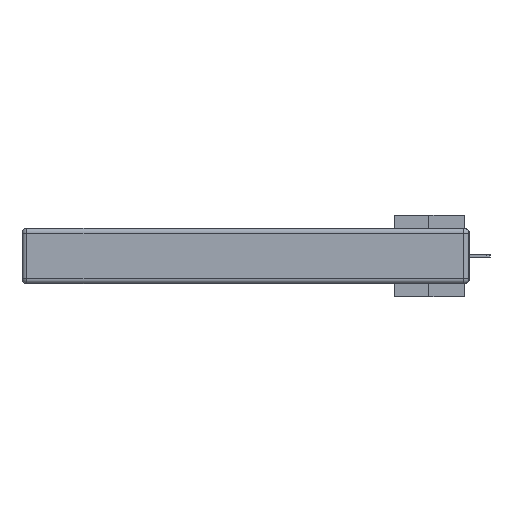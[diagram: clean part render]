
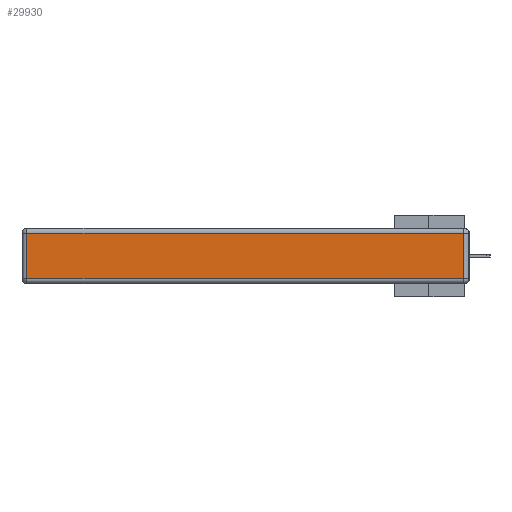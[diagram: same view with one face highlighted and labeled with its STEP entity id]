
A CAD part, left-side view. The second image highlights one B-rep face of the part: STEP entity #29930.
In plain terms, the highlighted planar face has unit normal (-1, 0, 0).
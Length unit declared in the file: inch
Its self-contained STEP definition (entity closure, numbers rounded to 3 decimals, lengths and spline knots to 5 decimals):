
#734 = LINE ( 'NONE', #21843, #33601 ) ;
#1146 = DIRECTION ( 'NONE',  ( 0., 0., -1. ) ) ;
#1558 = CARTESIAN_POINT ( 'NONE',  ( 0., 2.75, -0.03 ) ) ;
#3517 = EDGE_CURVE ( 'NONE', #15699, #11347, #24977, .T. ) ;
#5664 = EDGE_CURVE ( 'NONE', #13278, #15699, #734, .T. ) ;
#7889 = CARTESIAN_POINT ( 'NONE',  ( 0., 0.03, -0.313 ) ) ;
#8790 = EDGE_CURVE ( 'NONE', #21641, #13278, #31263, .T. ) ;
#10204 = DIRECTION ( 'NONE',  ( -1., 0., 0. ) ) ;
#11347 = VERTEX_POINT ( 'NONE', #38439 ) ;
#13143 = DIRECTION ( 'NONE',  ( 0., 0., 1. ) ) ;
#13278 = VERTEX_POINT ( 'NONE', #34834 ) ;
#13696 = PLANE ( 'NONE',  #26772 ) ;
#15699 = VERTEX_POINT ( 'NONE', #7889 ) ;
#16774 = CARTESIAN_POINT ( 'NONE',  ( 0., 0., -0.343 ) ) ;
#17540 = EDGE_LOOP ( 'NONE', ( #32841, #40774, #32799, #22112 ) ) ;
#20482 = CARTESIAN_POINT ( 'NONE',  ( 0., 2.72, -0.343 ) ) ;
#20594 = DIRECTION ( 'NONE',  ( 0., 1., 0. ) ) ;
#21641 = VERTEX_POINT ( 'NONE', #22743 ) ;
#21843 = CARTESIAN_POINT ( 'NONE',  ( 0., 0., -0.313 ) ) ;
#22112 = ORIENTED_EDGE ( 'NONE', *, *, #8790, .T. ) ;
#22632 = VECTOR ( 'NONE', #1146, 39.37008 ) ;
#22743 = CARTESIAN_POINT ( 'NONE',  ( 0., 2.72, -0.03 ) ) ;
#23723 = DIRECTION ( 'NONE',  ( 0., 0., 1. ) ) ;
#24672 = DIRECTION ( 'NONE',  ( 0., -1., 0. ) ) ;
#24851 = VECTOR ( 'NONE', #20594, 39.37008 ) ;
#24977 = LINE ( 'NONE', #36332, #41199 ) ;
#25193 = EDGE_CURVE ( 'NONE', #11347, #21641, #38025, .T. ) ;
#26772 = AXIS2_PLACEMENT_3D ( 'NONE', #16774, #10204, #13143 ) ;
#29930 = ADVANCED_FACE ( 'NONE', ( #41137 ), #13696, .T. ) ;
#31263 = LINE ( 'NONE', #20482, #22632 ) ;
#32799 = ORIENTED_EDGE ( 'NONE', *, *, #25193, .T. ) ;
#32841 = ORIENTED_EDGE ( 'NONE', *, *, #5664, .T. ) ;
#33601 = VECTOR ( 'NONE', #24672, 39.37008 ) ;
#34834 = CARTESIAN_POINT ( 'NONE',  ( 0., 2.72, -0.313 ) ) ;
#36332 = CARTESIAN_POINT ( 'NONE',  ( 0., 0.03, -0.343 ) ) ;
#38025 = LINE ( 'NONE', #1558, #24851 ) ;
#38439 = CARTESIAN_POINT ( 'NONE',  ( 0., 0.03, -0.03 ) ) ;
#40774 = ORIENTED_EDGE ( 'NONE', *, *, #3517, .T. ) ;
#41137 = FACE_OUTER_BOUND ( 'NONE', #17540, .T. ) ;
#41199 = VECTOR ( 'NONE', #23723, 39.37008 ) ;
